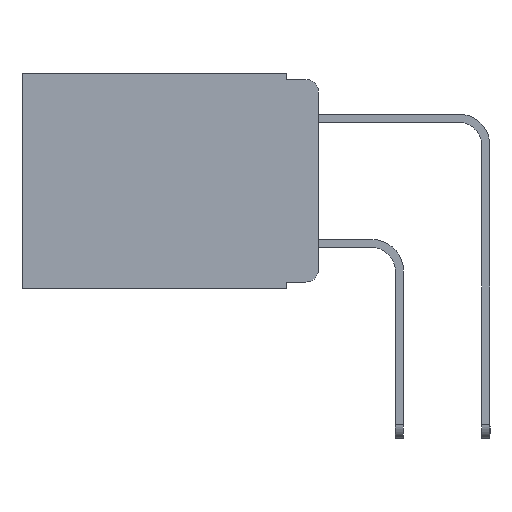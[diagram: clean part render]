
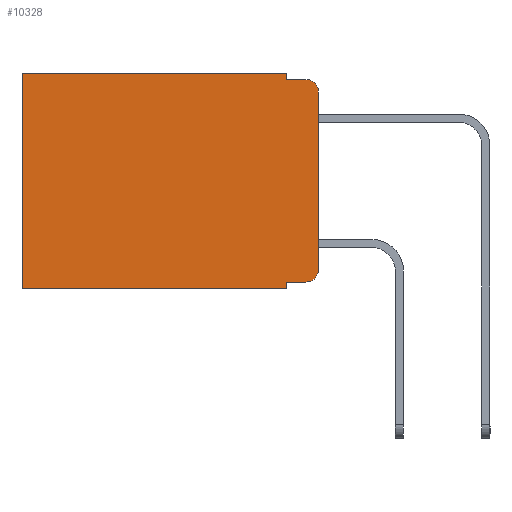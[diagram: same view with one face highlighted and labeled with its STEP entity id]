
A CAD part, left-side view. The second image highlights one B-rep face of the part: STEP entity #10328.
In plain terms, the highlighted planar face has unit normal (-1, 0, 0).
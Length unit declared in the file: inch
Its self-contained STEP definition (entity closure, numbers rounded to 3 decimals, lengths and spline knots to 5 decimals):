
#53 = ORIENTED_EDGE ( 'NONE', *, *, #5058, .F. ) ;
#245 = VECTOR ( 'NONE', #4906, 39.37008 ) ;
#467 = CARTESIAN_POINT ( 'NONE',  ( 0.298, 0.051, -0.343 ) ) ;
#543 = EDGE_CURVE ( 'NONE', #16230, #11727, #9895, .T. ) ;
#726 = AXIS2_PLACEMENT_3D ( 'NONE', #5993, #18374, #7769 ) ;
#761 = DIRECTION ( 'NONE',  ( 0., 0., -1. ) ) ;
#1026 = CARTESIAN_POINT ( 'NONE',  ( 0.298, 0.473, 0. ) ) ;
#1054 = ORIENTED_EDGE ( 'NONE', *, *, #543, .T. ) ;
#1291 = EDGE_CURVE ( 'NONE', #17165, #11727, #10344, .T. ) ;
#1374 = DIRECTION ( 'NONE',  ( 0., 1., 0. ) ) ;
#1628 = VERTEX_POINT ( 'NONE', #5756 ) ;
#2042 = CARTESIAN_POINT ( 'NONE',  ( 0.298, 0.02, -0.313 ) ) ;
#2206 = ORIENTED_EDGE ( 'NONE', *, *, #4085, .F. ) ;
#2305 = CARTESIAN_POINT ( 'NONE',  ( 0.298, 0.051, 0. ) ) ;
#2393 = LINE ( 'NONE', #2305, #7281 ) ;
#2573 = CARTESIAN_POINT ( 'NONE',  ( 0.298, 0.051, 0. ) ) ;
#3520 = CARTESIAN_POINT ( 'NONE',  ( 0.298, 0.02, -0.333 ) ) ;
#3670 = DIRECTION ( 'NONE',  ( 0., 0., -1. ) ) ;
#3722 = DIRECTION ( 'NONE',  ( 0., 0., -1. ) ) ;
#3898 = EDGE_CURVE ( 'NONE', #17165, #5739, #7274, .T. ) ;
#4006 = ORIENTED_EDGE ( 'NONE', *, *, #9239, .F. ) ;
#4085 = EDGE_CURVE ( 'NONE', #14084, #8020, #17110, .T. ) ;
#4603 = CARTESIAN_POINT ( 'NONE',  ( 0.298, 0.051, -0.01 ) ) ;
#4794 = CARTESIAN_POINT ( 'NONE',  ( 0.298, 0.051, -0.333 ) ) ;
#4906 = DIRECTION ( 'NONE',  ( 0., 0., -1. ) ) ;
#5058 = EDGE_CURVE ( 'NONE', #8690, #14084, #13929, .T. ) ;
#5406 = VERTEX_POINT ( 'NONE', #1026 ) ;
#5460 = ORIENTED_EDGE ( 'NONE', *, *, #1291, .F. ) ;
#5552 = CARTESIAN_POINT ( 'NONE',  ( 0.298, 0.051, 0. ) ) ;
#5739 = VERTEX_POINT ( 'NONE', #7862 ) ;
#5756 = CARTESIAN_POINT ( 'NONE',  ( 0.298, 0.051, -0.01 ) ) ;
#5993 = CARTESIAN_POINT ( 'NONE',  ( 0.298, 0.02, -0.03 ) ) ;
#7119 = VECTOR ( 'NONE', #15086, 39.37008 ) ;
#7225 = FACE_OUTER_BOUND ( 'NONE', #16526, .T. ) ;
#7274 = CIRCLE ( 'NONE', #726, 0.02 ) ;
#7281 = VECTOR ( 'NONE', #3670, 39.37008 ) ;
#7462 = CARTESIAN_POINT ( 'NONE',  ( 0.298, 0., 0. ) ) ;
#7769 = DIRECTION ( 'NONE',  ( 0., 0., -1. ) ) ;
#7862 = CARTESIAN_POINT ( 'NONE',  ( 0.298, 0.02, -0.01 ) ) ;
#7905 = VECTOR ( 'NONE', #13823, 39.37008 ) ;
#7983 = EDGE_CURVE ( 'NONE', #8690, #16230, #14884, .T. ) ;
#8015 = VECTOR ( 'NONE', #1374, 39.37008 ) ;
#8020 = VERTEX_POINT ( 'NONE', #9326 ) ;
#8184 = ORIENTED_EDGE ( 'NONE', *, *, #7983, .T. ) ;
#8622 = AXIS2_PLACEMENT_3D ( 'NONE', #13330, #18924, #17840 ) ;
#8650 = CARTESIAN_POINT ( 'NONE',  ( 0.298, 0., 0. ) ) ;
#8690 = VERTEX_POINT ( 'NONE', #4794 ) ;
#8890 = ORIENTED_EDGE ( 'NONE', *, *, #8937, .T. ) ;
#8937 = EDGE_CURVE ( 'NONE', #5406, #8020, #15482, .T. ) ;
#9235 = LINE ( 'NONE', #4603, #7119 ) ;
#9239 = EDGE_CURVE ( 'NONE', #18956, #1628, #2393, .T. ) ;
#9326 = CARTESIAN_POINT ( 'NONE',  ( 0.298, 0.473, -0.343 ) ) ;
#9767 = CARTESIAN_POINT ( 'NONE',  ( 0.298, 0., -0.343 ) ) ;
#9895 = CIRCLE ( 'NONE', #14324, 0.02 ) ;
#10141 = VECTOR ( 'NONE', #3722, 39.37008 ) ;
#10328 = ADVANCED_FACE ( 'NONE', ( #7225 ), #13239, .F. ) ;
#10344 = LINE ( 'NONE', #7462, #245 ) ;
#10774 = CARTESIAN_POINT ( 'NONE',  ( 0.298, 0.051, -0.333 ) ) ;
#10903 = DIRECTION ( 'NONE',  ( 0., 0., -1. ) ) ;
#11186 = CARTESIAN_POINT ( 'NONE',  ( 0.298, 0.473, 0. ) ) ;
#11727 = VERTEX_POINT ( 'NONE', #16660 ) ;
#12794 = ORIENTED_EDGE ( 'NONE', *, *, #14824, .F. ) ;
#12975 = LINE ( 'NONE', #8650, #8015 ) ;
#13239 = PLANE ( 'NONE',  #8622 ) ;
#13330 = CARTESIAN_POINT ( 'NONE',  ( 0.298, 0., 0. ) ) ;
#13356 = EDGE_CURVE ( 'NONE', #18956, #5406, #12975, .T. ) ;
#13823 = DIRECTION ( 'NONE',  ( 0., -1., 0. ) ) ;
#13929 = LINE ( 'NONE', #5552, #14865 ) ;
#14084 = VERTEX_POINT ( 'NONE', #467 ) ;
#14324 = AXIS2_PLACEMENT_3D ( 'NONE', #2042, #15669, #761 ) ;
#14824 = EDGE_CURVE ( 'NONE', #1628, #5739, #9235, .T. ) ;
#14865 = VECTOR ( 'NONE', #10903, 39.37008 ) ;
#14884 = LINE ( 'NONE', #10774, #7905 ) ;
#15086 = DIRECTION ( 'NONE',  ( 0., -1., 0. ) ) ;
#15482 = LINE ( 'NONE', #11186, #10141 ) ;
#15669 = DIRECTION ( 'NONE',  ( -1., 0., 0. ) ) ;
#15731 = DIRECTION ( 'NONE',  ( 0., 1., 0. ) ) ;
#16230 = VERTEX_POINT ( 'NONE', #3520 ) ;
#16526 = EDGE_LOOP ( 'NONE', ( #5460, #16971, #12794, #4006, #17243, #8890, #2206, #53, #8184, #1054 ) ) ;
#16660 = CARTESIAN_POINT ( 'NONE',  ( 0.298, 0., -0.313 ) ) ;
#16946 = CARTESIAN_POINT ( 'NONE',  ( 0.298, 0., -0.03 ) ) ;
#16971 = ORIENTED_EDGE ( 'NONE', *, *, #3898, .T. ) ;
#17066 = VECTOR ( 'NONE', #15731, 39.37008 ) ;
#17110 = LINE ( 'NONE', #9767, #17066 ) ;
#17165 = VERTEX_POINT ( 'NONE', #16946 ) ;
#17243 = ORIENTED_EDGE ( 'NONE', *, *, #13356, .T. ) ;
#17840 = DIRECTION ( 'NONE',  ( 0., 0., -1. ) ) ;
#18374 = DIRECTION ( 'NONE',  ( -1., 0., 0. ) ) ;
#18924 = DIRECTION ( 'NONE',  ( 1., 0., 0. ) ) ;
#18956 = VERTEX_POINT ( 'NONE', #2573 ) ;
